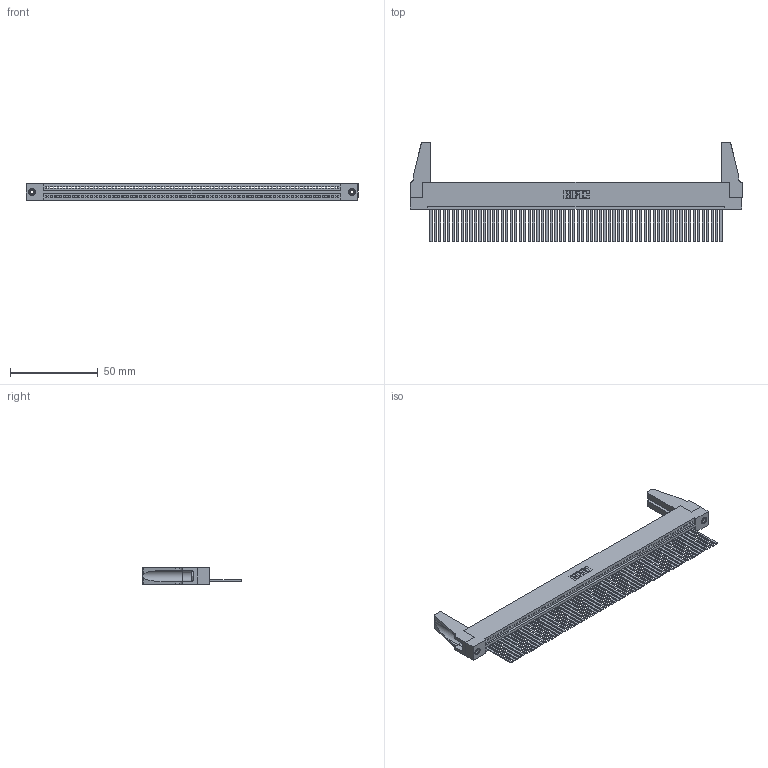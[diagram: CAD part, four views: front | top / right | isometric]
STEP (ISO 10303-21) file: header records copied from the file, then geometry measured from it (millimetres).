
FILE_DESCRIPTION (( 'STEP AP203' ), '1' );
FILE_NAME ('395-066-544-188.STEP', '2019-10-25T09:44:32', ( '' ), ( '' ), 'SwSTEP 2.0', 'SolidWorks 2016', '' );
FILE_SCHEMA (( 'CONFIG_CONTROL_DESIGN' ));
Length unit declared in the file: inch
Products named in the file (5): 345 Part_Flush Mounting Lugs - 0.156 Dia-TH; 345-220-078_345-220-088; 345-292-001_345-293-144; 395-066-544-188; 345-250-001_345-250-001-102
Assembly tree (71 placements, depth 2):
  395-066-544-188
    345 Part_Flush Mounting Lugs - 0.156 Dia-TH
    345-292-001_345-293-144  x66
    345-250-001_345-250-001-102  x2
    345-220-078_345-220-088  x2
Bounding box: 188.87 x 56.82 x 9.4 mm (x, y, z)
Volume: 22152.9 mm3; surface area: 30867.1 mm2
Topology: 71 solids, 71 shells, 3682 faces, 11083 edges, 7290 vertices
Faces by surface type: plane 2528, cylinder 1138, cone 12, torus 4
Entity records: 48406 total; most frequent: CARTESIAN_POINT 8372, ORIENTED_EDGE 8332, DIRECTION 7282, EDGE_CURVE 4166, VECTOR 3732, LINE 3732, VERTEX_POINT 2770, AXIS2_PLACEMENT_3D 1775
